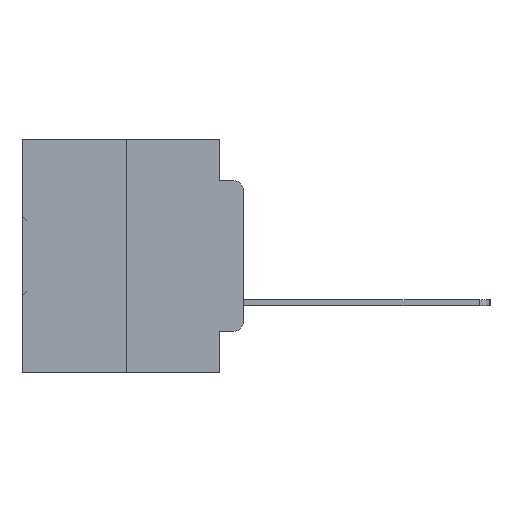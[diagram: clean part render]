
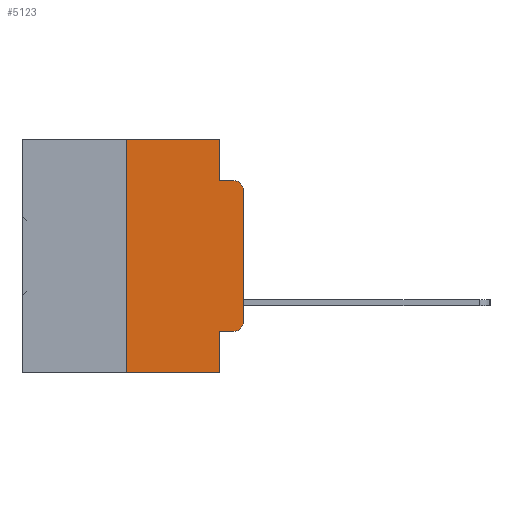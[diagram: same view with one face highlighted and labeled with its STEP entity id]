
A CAD part, left-side view. The second image highlights one B-rep face of the part: STEP entity #5123.
In plain terms, the highlighted planar face has unit normal (-1, 0, 0).
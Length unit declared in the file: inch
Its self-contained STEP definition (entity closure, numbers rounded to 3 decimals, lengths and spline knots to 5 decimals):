
#264 = CARTESIAN_POINT ( 'NONE',  ( 0., 0.051, -0.0885 ) ) ;
#1981 = VECTOR ( 'NONE', #12471, 39.37008 ) ;
#2568 = DIRECTION ( 'NONE',  ( 0., -1., 0. ) ) ;
#2800 = AXIS2_PLACEMENT_3D ( 'NONE', #26835, #10159, #29624 ) ;
#3114 = VERTEX_POINT ( 'NONE', #10276 ) ;
#3167 = EDGE_CURVE ( 'NONE', #22541, #13736, #11474, .T. ) ;
#3359 = ORIENTED_EDGE ( 'NONE', *, *, #14542, .T. ) ;
#3414 = VERTEX_POINT ( 'NONE', #8662 ) ;
#3944 = DIRECTION ( 'NONE',  ( 0., 0., -1. ) ) ;
#4186 = CARTESIAN_POINT ( 'NONE',  ( 0., 0., -0.1085 ) ) ;
#4665 = CARTESIAN_POINT ( 'NONE',  ( 0., 0.25, 0. ) ) ;
#4927 = LINE ( 'NONE', #21355, #25499 ) ;
#5008 = CARTESIAN_POINT ( 'NONE',  ( 0., 0.473, -0.5 ) ) ;
#5100 = EDGE_CURVE ( 'NONE', #5331, #15307, #30057, .T. ) ;
#5123 = ADVANCED_FACE ( 'NONE', ( #7859 ), #6085, .F. ) ;
#5331 = VERTEX_POINT ( 'NONE', #15521 ) ;
#5629 = ORIENTED_EDGE ( 'NONE', *, *, #28258, .T. ) ;
#6079 = ORIENTED_EDGE ( 'NONE', *, *, #24133, .F. ) ;
#6085 = PLANE ( 'NONE',  #7665 ) ;
#6516 = EDGE_LOOP ( 'NONE', ( #16609, #3359, #25717, #20089, #6079, #22697, #8743, #25310, #32636, #5629 ) ) ;
#7049 = EDGE_CURVE ( 'NONE', #15307, #35838, #33362, .T. ) ;
#7665 = AXIS2_PLACEMENT_3D ( 'NONE', #28383, #11707, #31158 ) ;
#7859 = FACE_OUTER_BOUND ( 'NONE', #6516, .T. ) ;
#8582 = CARTESIAN_POINT ( 'NONE',  ( 0., 0.02, -0.0885 ) ) ;
#8662 = CARTESIAN_POINT ( 'NONE',  ( 0., 0.02, -0.4115 ) ) ;
#8743 = ORIENTED_EDGE ( 'NONE', *, *, #20624, .T. ) ;
#8792 = CIRCLE ( 'NONE', #15312, 0.02 ) ;
#9607 = LINE ( 'NONE', #5008, #23562 ) ;
#10159 = DIRECTION ( 'NONE',  ( -1., 0., 0. ) ) ;
#10276 = CARTESIAN_POINT ( 'NONE',  ( 0., 0.051, -0.5 ) ) ;
#10504 = DIRECTION ( 'NONE',  ( -1., 0., 0. ) ) ;
#11474 = LINE ( 'NONE', #18829, #25422 ) ;
#11707 = DIRECTION ( 'NONE',  ( 1., 0., 0. ) ) ;
#12068 = CARTESIAN_POINT ( 'NONE',  ( 0., 0., -0.3915 ) ) ;
#12118 = VECTOR ( 'NONE', #17233, 39.37008 ) ;
#12471 = DIRECTION ( 'NONE',  ( 0., -1., 0. ) ) ;
#13372 = CARTESIAN_POINT ( 'NONE',  ( 0., 0.051, -0.4115 ) ) ;
#13434 = CARTESIAN_POINT ( 'NONE',  ( 0., 0.051, 0. ) ) ;
#13736 = VERTEX_POINT ( 'NONE', #4665 ) ;
#14542 = EDGE_CURVE ( 'NONE', #21124, #35838, #22625, .T. ) ;
#15284 = VECTOR ( 'NONE', #24637, 39.37008 ) ;
#15307 = VERTEX_POINT ( 'NONE', #16112 ) ;
#15312 = AXIS2_PLACEMENT_3D ( 'NONE', #27170, #10504, #29949 ) ;
#15521 = CARTESIAN_POINT ( 'NONE',  ( 0., 0.051, 0. ) ) ;
#16112 = CARTESIAN_POINT ( 'NONE',  ( 0., 0.051, -0.0885 ) ) ;
#16435 = EDGE_CURVE ( 'NONE', #19077, #21124, #4927, .T. ) ;
#16609 = ORIENTED_EDGE ( 'NONE', *, *, #16435, .T. ) ;
#17233 = DIRECTION ( 'NONE',  ( 0., -1., 0. ) ) ;
#18829 = CARTESIAN_POINT ( 'NONE',  ( 0., 0.25, 0. ) ) ;
#19077 = VERTEX_POINT ( 'NONE', #12068 ) ;
#20089 = ORIENTED_EDGE ( 'NONE', *, *, #5100, .F. ) ;
#20624 = EDGE_CURVE ( 'NONE', #22541, #3114, #9607, .T. ) ;
#21124 = VERTEX_POINT ( 'NONE', #4186 ) ;
#21355 = CARTESIAN_POINT ( 'NONE',  ( 0., 0., 0. ) ) ;
#21594 = DIRECTION ( 'NONE',  ( 0., 0., 1. ) ) ;
#22541 = VERTEX_POINT ( 'NONE', #33335 ) ;
#22625 = CIRCLE ( 'NONE', #2800, 0.02 ) ;
#22697 = ORIENTED_EDGE ( 'NONE', *, *, #3167, .F. ) ;
#23562 = VECTOR ( 'NONE', #27390, 39.37008 ) ;
#23897 = LINE ( 'NONE', #26355, #1981 ) ;
#24133 = EDGE_CURVE ( 'NONE', #13736, #5331, #33189, .T. ) ;
#24157 = DIRECTION ( 'NONE',  ( 0., 0., 1. ) ) ;
#24637 = DIRECTION ( 'NONE',  ( 0., 0., -1. ) ) ;
#25025 = VECTOR ( 'NONE', #2568, 39.37008 ) ;
#25310 = ORIENTED_EDGE ( 'NONE', *, *, #31962, .F. ) ;
#25422 = VECTOR ( 'NONE', #21594, 39.37008 ) ;
#25499 = VECTOR ( 'NONE', #24157, 39.37008 ) ;
#25717 = ORIENTED_EDGE ( 'NONE', *, *, #7049, .F. ) ;
#25774 = LINE ( 'NONE', #29037, #33087 ) ;
#26355 = CARTESIAN_POINT ( 'NONE',  ( 0., 0.051, -0.4115 ) ) ;
#26835 = CARTESIAN_POINT ( 'NONE',  ( 0., 0.02, -0.1085 ) ) ;
#27170 = CARTESIAN_POINT ( 'NONE',  ( 0., 0.02, -0.3915 ) ) ;
#27390 = DIRECTION ( 'NONE',  ( 0., -1., 0. ) ) ;
#28258 = EDGE_CURVE ( 'NONE', #3414, #19077, #8792, .T. ) ;
#28383 = CARTESIAN_POINT ( 'NONE',  ( 0., 0.473, 0. ) ) ;
#29037 = CARTESIAN_POINT ( 'NONE',  ( 0., 0.051, 0. ) ) ;
#29624 = DIRECTION ( 'NONE',  ( 0., 0., -1. ) ) ;
#29949 = DIRECTION ( 'NONE',  ( 0., 0., -1. ) ) ;
#30057 = LINE ( 'NONE', #13434, #15284 ) ;
#30135 = EDGE_CURVE ( 'NONE', #31495, #3414, #23897, .T. ) ;
#31158 = DIRECTION ( 'NONE',  ( 0., 0., -1. ) ) ;
#31495 = VERTEX_POINT ( 'NONE', #13372 ) ;
#31962 = EDGE_CURVE ( 'NONE', #31495, #3114, #25774, .T. ) ;
#32636 = ORIENTED_EDGE ( 'NONE', *, *, #30135, .T. ) ;
#33087 = VECTOR ( 'NONE', #3944, 39.37008 ) ;
#33189 = LINE ( 'NONE', #35942, #25025 ) ;
#33335 = CARTESIAN_POINT ( 'NONE',  ( 0., 0.25, -0.5 ) ) ;
#33362 = LINE ( 'NONE', #264, #12118 ) ;
#35838 = VERTEX_POINT ( 'NONE', #8582 ) ;
#35942 = CARTESIAN_POINT ( 'NONE',  ( 0., 0.473, 0. ) ) ;
